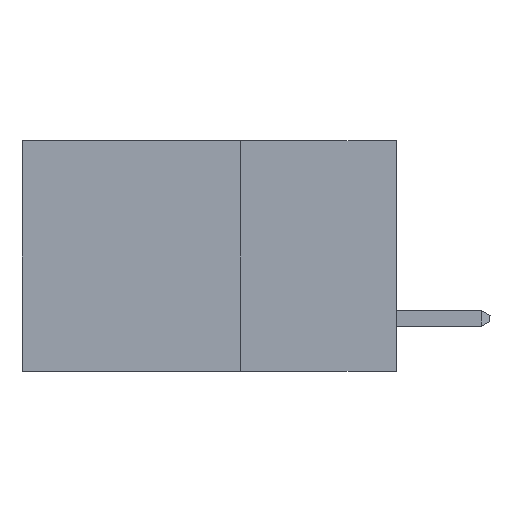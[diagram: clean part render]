
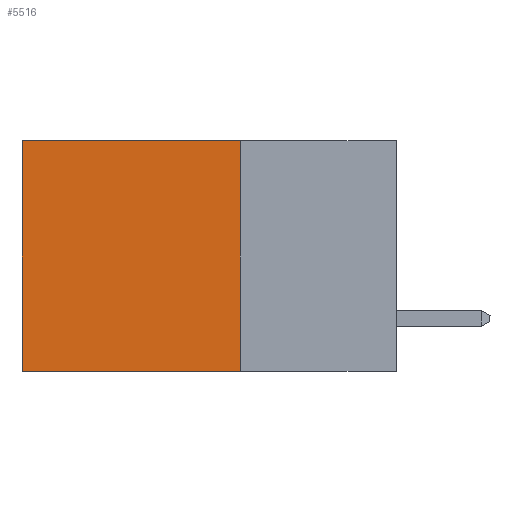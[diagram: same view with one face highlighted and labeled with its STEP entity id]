
A CAD part, left-side view. The second image highlights one B-rep face of the part: STEP entity #5516.
In plain terms, the highlighted planar face has unit normal (-1, 0, 0).
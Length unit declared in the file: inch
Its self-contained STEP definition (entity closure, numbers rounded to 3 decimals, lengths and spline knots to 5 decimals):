
#241 = LINE ( 'NONE', #2157, #19758 ) ;
#1220 = CARTESIAN_POINT ( 'NONE',  ( 0.2615, 0.25, 0. ) ) ;
#1715 = DIRECTION ( 'NONE',  ( 0., 1., 0. ) ) ;
#1978 = EDGE_CURVE ( 'NONE', #18265, #11169, #241, .T. ) ;
#2140 = CARTESIAN_POINT ( 'NONE',  ( 0.2615, 0.25, -0.37 ) ) ;
#2157 = CARTESIAN_POINT ( 'NONE',  ( 0.2615, 0.25, -0.37 ) ) ;
#4084 = VECTOR ( 'NONE', #4131, 39.37008 ) ;
#4089 = DIRECTION ( 'NONE',  ( 0., 0., -1. ) ) ;
#4131 = DIRECTION ( 'NONE',  ( 0., 0., -1. ) ) ;
#4262 = CARTESIAN_POINT ( 'NONE',  ( 0.2615, 0.6, -0.37 ) ) ;
#4905 = DIRECTION ( 'NONE',  ( 0., 1., 0. ) ) ;
#4999 = FACE_OUTER_BOUND ( 'NONE', #8367, .T. ) ;
#5084 = LINE ( 'NONE', #2140, #14534 ) ;
#5516 = ADVANCED_FACE ( 'NONE', ( #4999 ), #11697, .F. ) ;
#6103 = CARTESIAN_POINT ( 'NONE',  ( 0.2615, 0.6, 0. ) ) ;
#6202 = EDGE_CURVE ( 'NONE', #19653, #11169, #9679, .T. ) ;
#6409 = LINE ( 'NONE', #24074, #20755 ) ;
#7304 = VERTEX_POINT ( 'NONE', #1220 ) ;
#8004 = EDGE_CURVE ( 'NONE', #7304, #19653, #6409, .T. ) ;
#8367 = EDGE_LOOP ( 'NONE', ( #23721, #11632, #13041, #18659 ) ) ;
#9679 = LINE ( 'NONE', #4262, #4084 ) ;
#10724 = CARTESIAN_POINT ( 'NONE',  ( 0.2615, 0.6, -0.37 ) ) ;
#11169 = VERTEX_POINT ( 'NONE', #10724 ) ;
#11590 = DIRECTION ( 'NONE',  ( 0., 0., -1. ) ) ;
#11613 = DIRECTION ( 'NONE',  ( 1., 0., 0. ) ) ;
#11632 = ORIENTED_EDGE ( 'NONE', *, *, #1978, .F. ) ;
#11663 = CARTESIAN_POINT ( 'NONE',  ( 0.2615, 0.25, -0.37 ) ) ;
#11697 = PLANE ( 'NONE',  #12179 ) ;
#12179 = AXIS2_PLACEMENT_3D ( 'NONE', #11663, #11613, #11590 ) ;
#13041 = ORIENTED_EDGE ( 'NONE', *, *, #20107, .F. ) ;
#14534 = VECTOR ( 'NONE', #4089, 39.37008 ) ;
#16690 = CARTESIAN_POINT ( 'NONE',  ( 0.2615, 0.25, -0.37 ) ) ;
#18265 = VERTEX_POINT ( 'NONE', #16690 ) ;
#18659 = ORIENTED_EDGE ( 'NONE', *, *, #8004, .T. ) ;
#19653 = VERTEX_POINT ( 'NONE', #6103 ) ;
#19758 = VECTOR ( 'NONE', #4905, 39.37008 ) ;
#20107 = EDGE_CURVE ( 'NONE', #7304, #18265, #5084, .T. ) ;
#20755 = VECTOR ( 'NONE', #1715, 39.37008 ) ;
#23721 = ORIENTED_EDGE ( 'NONE', *, *, #6202, .T. ) ;
#24074 = CARTESIAN_POINT ( 'NONE',  ( 0.2615, 0.25, 0. ) ) ;
